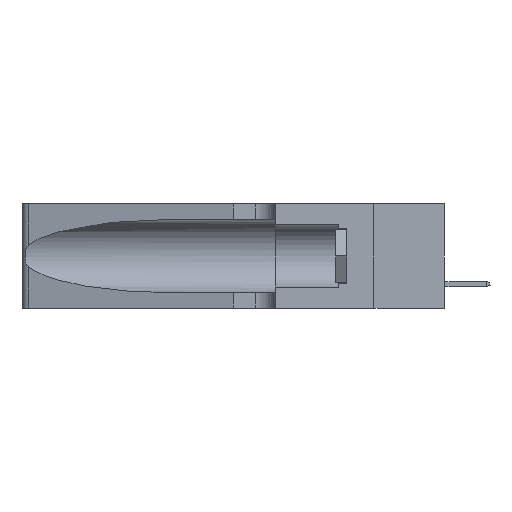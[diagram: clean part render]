
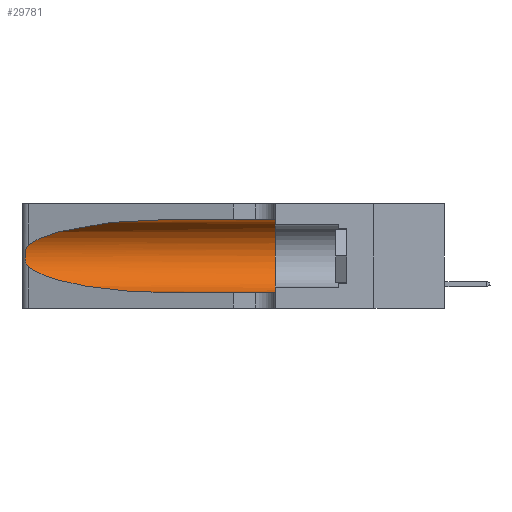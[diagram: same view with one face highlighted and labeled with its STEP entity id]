
A CAD part, left-side view. The second image highlights one B-rep face of the part: STEP entity #29781.
In plain terms, the highlighted cylindrical face has radius 3.308 mm (diameter 6.617 mm), a partial arc.
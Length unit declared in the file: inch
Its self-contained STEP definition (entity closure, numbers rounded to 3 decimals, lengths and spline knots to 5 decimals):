
#318 = VECTOR ( 'NONE', #45157, 39.37008 ) ;
#577 = CARTESIAN_POINT ( 'NONE',  ( 0.1305, 0.35, 0.05475 ) ) ;
#925 = CARTESIAN_POINT ( 'NONE',  ( 0.26075, 1.23896, 0.19203 ) ) ;
#1571 = ORIENTED_EDGE ( 'NONE', *, *, #38637, .T. ) ;
#3397 = CARTESIAN_POINT ( 'NONE',  ( 0.1305, 0.72297, 0.05475 ) ) ;
#3435 = CARTESIAN_POINT ( 'NONE',  ( 0.1305, 0.72297, 0.31525 ) ) ;
#3534 = CARTESIAN_POINT ( 'NONE',  ( 0.25487, 1.22718, 0.22369 ) ) ;
#4123 = VECTOR ( 'NONE', #41701, 39.37008 ) ;
#5508 = DIRECTION ( 'NONE',  ( 0., -1., 0. ) ) ;
#6039 = CARTESIAN_POINT ( 'NONE',  ( 0.25639, 1.23184, 0.21858 ) ) ;
#7549 = VERTEX_POINT ( 'NONE', #18035 ) ;
#7575 = CARTESIAN_POINT ( 'NONE',  ( 0.2373, 1.15595, 0.08982 ) ) ;
#7904 = CARTESIAN_POINT ( 'NONE',  ( 0.2373, 1.15595, 0.28018 ) ) ;
#8191 = AXIS2_PLACEMENT_3D ( 'NONE', #21570, #48605, #18862 ) ;
#11876 = CIRCLE ( 'NONE', #8191, 0.13025 ) ;
#12878 = VERTEX_POINT ( 'NONE', #47694 ) ;
#13810 = CARTESIAN_POINT ( 'NONE',  ( 0.1305, 0.35, 0.31525 ) ) ;
#14905 = CARTESIAN_POINT ( 'NONE',  ( 0.1305, 1.61858, 0.31525 ) ) ;
#15519 = CYLINDRICAL_SURFACE ( 'NONE', #27299, 0.13025 ) ;
#16738 = CARTESIAN_POINT ( 'NONE',  ( 0.25555, 1.22993, 0.14849 ) ) ;
#17178 = ORIENTED_EDGE ( 'NONE', *, *, #35597, .T. ) ;
#18035 = CARTESIAN_POINT ( 'NONE',  ( 0.1305, 0.72297, 0.05475 ) ) ;
#18862 = DIRECTION ( 'NONE',  ( 0., 0., 1. ) ) ;
#18996 = CARTESIAN_POINT ( 'NONE',  ( 0.25487, 1.22718, 0.22369 ) ) ;
#19487 = EDGE_LOOP ( 'NONE', ( #44605, #22955, #17178, #1571, #41342, #20977 ) ) ;
#20977 = ORIENTED_EDGE ( 'NONE', *, *, #49464, .F. ) ;
#21570 = CARTESIAN_POINT ( 'NONE',  ( 0.1305, 0.35, 0.185 ) ) ;
#21728 = VERTEX_POINT ( 'NONE', #3534 ) ;
#22383 = CARTESIAN_POINT ( 'NONE',  ( 0.18966, 0.96281, 0.05475 ) ) ;
#22955 = ORIENTED_EDGE ( 'NONE', *, *, #24088, .T. ) ;
#23999 = CARTESIAN_POINT ( 'NONE',  ( 0.26075, 1.23896, 0.178 ) ) ;
#24088 = EDGE_CURVE ( 'NONE', #21728, #12878, #44402, .T. ) ;
#24301 = CARTESIAN_POINT ( 'NONE',  ( 0.1305, 0.72297, 0.31525 ) ) ;
#24900 =( BOUNDED_CURVE ( )  B_SPLINE_CURVE ( 3, ( #3435, #42475, #7904, #18996 ),
 .UNSPECIFIED., .F., .F. ) 
 B_SPLINE_CURVE_WITH_KNOTS ( ( 4, 4 ),
 ( 1.5708, 2.84003 ),
 .UNSPECIFIED. ) 
 CURVE ( )  GEOMETRIC_REPRESENTATION_ITEM ( )  RATIONAL_B_SPLINE_CURVE ( ( 1., 0.87, 0.87, 1. ) ) 
 REPRESENTATION_ITEM ( '' )  );
#26664 = CARTESIAN_POINT ( 'NONE',  ( 0.25789, 1.23486, 0.15765 ) ) ;
#27299 = AXIS2_PLACEMENT_3D ( 'NONE', #27526, #5508, #32440 ) ;
#27526 = CARTESIAN_POINT ( 'NONE',  ( 0.1305, 1.61858, 0.185 ) ) ;
#29531 = CARTESIAN_POINT ( 'NONE',  ( 0.1305, 1.61858, 0.05475 ) ) ;
#29656 = CARTESIAN_POINT ( 'NONE',  ( 0.26017, 1.23833, 0.17102 ) ) ;
#29781 = ADVANCED_FACE ( 'NONE', ( #45816 ), #15519, .F. ) ;
#32440 = DIRECTION ( 'NONE',  ( 0., 0., -1. ) ) ;
#35597 = EDGE_CURVE ( 'NONE', #12878, #7549, #43445, .T. ) ;
#35947 = VERTEX_POINT ( 'NONE', #577 ) ;
#38535 = CARTESIAN_POINT ( 'NONE',  ( 0.25787, 1.23484, 0.2124 ) ) ;
#38590 = EDGE_CURVE ( 'NONE', #39887, #35947, #11876, .T. ) ;
#38637 = EDGE_CURVE ( 'NONE', #7549, #35947, #40265, .T. ) ;
#38712 = EDGE_CURVE ( 'NONE', #45219, #21728, #24900, .T. ) ;
#39887 = VERTEX_POINT ( 'NONE', #13810 ) ;
#39968 = CARTESIAN_POINT ( 'NONE',  ( 0.25856, 1.23593, 0.16098 ) ) ;
#40265 = LINE ( 'NONE', #29531, #4123 ) ;
#40743 = CARTESIAN_POINT ( 'NONE',  ( 0.25487, 1.22718, 0.22369 ) ) ;
#40864 = CARTESIAN_POINT ( 'NONE',  ( 0.25854, 1.2359, 0.20912 ) ) ;
#41342 = ORIENTED_EDGE ( 'NONE', *, *, #38590, .F. ) ;
#41701 = DIRECTION ( 'NONE',  ( 0., -1., 0. ) ) ;
#42475 = CARTESIAN_POINT ( 'NONE',  ( 0.18966, 0.96281, 0.31525 ) ) ;
#43445 =( BOUNDED_CURVE ( )  B_SPLINE_CURVE ( 3, ( #49897, #7575, #22383, #3397 ),
 .UNSPECIFIED., .F., .T. ) 
 B_SPLINE_CURVE_WITH_KNOTS ( ( 4, 4 ),
 ( 3.44316, 4.71239 ),
 .UNSPECIFIED. ) 
 CURVE ( )  GEOMETRIC_REPRESENTATION_ITEM ( )  RATIONAL_B_SPLINE_CURVE ( ( 1., 0.87, 0.87, 1. ) ) 
 REPRESENTATION_ITEM ( '' )  );
#44300 = CARTESIAN_POINT ( 'NONE',  ( 0.25639, 1.23186, 0.15144 ) ) ;
#44334 = LINE ( 'NONE', #14905, #318 ) ;
#44402 = B_SPLINE_CURVE_WITH_KNOTS ( 'NONE', 3,
 ( #40743, #48125, #6039, #38535, #40864, #44751, #925, #23999, #29656, #39968, #26664, #44300, #16738, #47204 ),
 .UNSPECIFIED., .F., .F.,
 ( 4, 2, 2, 2, 2, 2, 4 ),
 ( 0., 0.00027, 0.00053, 0.00107, 0.0016, 0.00187, 0.00214 ),
 .UNSPECIFIED. ) ;
#44605 = ORIENTED_EDGE ( 'NONE', *, *, #38712, .T. ) ;
#44751 = CARTESIAN_POINT ( 'NONE',  ( 0.26018, 1.23835, 0.19895 ) ) ;
#45157 = DIRECTION ( 'NONE',  ( 0., -1., 0. ) ) ;
#45219 = VERTEX_POINT ( 'NONE', #24301 ) ;
#45816 = FACE_OUTER_BOUND ( 'NONE', #19487, .T. ) ;
#47204 = CARTESIAN_POINT ( 'NONE',  ( 0.25487, 1.22718, 0.14631 ) ) ;
#47694 = CARTESIAN_POINT ( 'NONE',  ( 0.25487, 1.22718, 0.14631 ) ) ;
#48125 = CARTESIAN_POINT ( 'NONE',  ( 0.25555, 1.22994, 0.2215 ) ) ;
#48605 = DIRECTION ( 'NONE',  ( 0., 1., 0. ) ) ;
#49464 = EDGE_CURVE ( 'NONE', #45219, #39887, #44334, .T. ) ;
#49897 = CARTESIAN_POINT ( 'NONE',  ( 0.25487, 1.22718, 0.14631 ) ) ;
